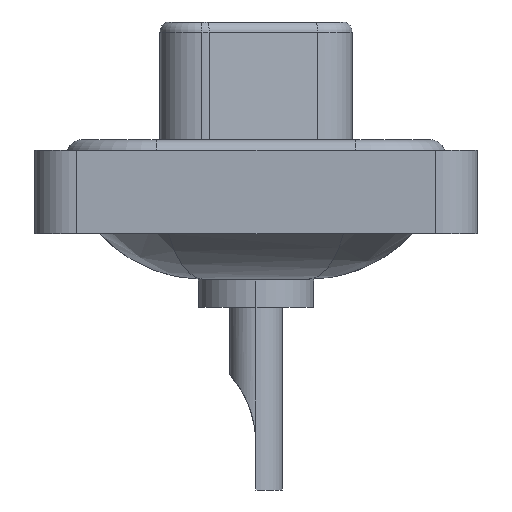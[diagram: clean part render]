
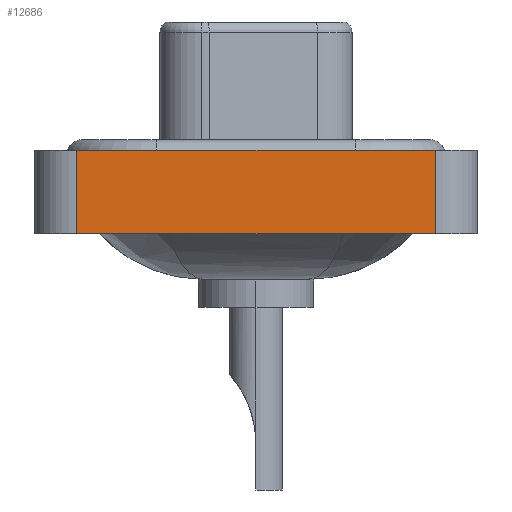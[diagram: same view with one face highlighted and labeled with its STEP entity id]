
A CAD part, left-side view. The second image highlights one B-rep face of the part: STEP entity #12686.
In plain terms, the highlighted planar face has unit normal (-1, 0, 0).
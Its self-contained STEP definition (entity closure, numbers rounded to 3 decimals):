
#684 = EDGE_CURVE ( 'NONE', #8553, #4325, #3760, .T. ) ;
#917 = EDGE_CURVE ( 'NONE', #8553, #6550, #10787, .T. ) ;
#930 = ORIENTED_EDGE ( 'NONE', *, *, #1071, .F. ) ;
#1071 = EDGE_CURVE ( 'NONE', #6550, #2067, #12765, .T. ) ;
#1132 = VECTOR ( 'NONE', #14625, 1000. ) ;
#2000 = CARTESIAN_POINT ( 'NONE',  ( -7.25, -8.55, 0.4 ) ) ;
#2067 = VERTEX_POINT ( 'NONE', #7733 ) ;
#2398 = AXIS2_PLACEMENT_3D ( 'NONE', #4824, #15515, #7355 ) ;
#2834 = LINE ( 'NONE', #7643, #1132 ) ;
#3626 = CARTESIAN_POINT ( 'NONE',  ( -7.25, 8.55, -3.6 ) ) ;
#3704 = DIRECTION ( 'NONE',  ( 0., 0., 1. ) ) ;
#3760 = LINE ( 'NONE', #14757, #11180 ) ;
#3839 = DIRECTION ( 'NONE',  ( 0., -1., 0. ) ) ;
#4325 = VERTEX_POINT ( 'NONE', #8404 ) ;
#4824 = CARTESIAN_POINT ( 'NONE',  ( -7.25, -8.55, -3.6 ) ) ;
#4906 = PLANE ( 'NONE',  #2398 ) ;
#6006 = FACE_OUTER_BOUND ( 'NONE', #14473, .T. ) ;
#6550 = VERTEX_POINT ( 'NONE', #6688 ) ;
#6558 = ORIENTED_EDGE ( 'NONE', *, *, #7739, .T. ) ;
#6688 = CARTESIAN_POINT ( 'NONE',  ( -7.25, 8.55, 0.4 ) ) ;
#6800 = DIRECTION ( 'NONE',  ( 0., -1., 0. ) ) ;
#6931 = ORIENTED_EDGE ( 'NONE', *, *, #917, .F. ) ;
#7131 = CARTESIAN_POINT ( 'NONE',  ( -7.25, 8.55, -3.6 ) ) ;
#7355 = DIRECTION ( 'NONE',  ( 0., 0., 1. ) ) ;
#7643 = CARTESIAN_POINT ( 'NONE',  ( -7.25, -8.55, -3.6 ) ) ;
#7733 = CARTESIAN_POINT ( 'NONE',  ( -7.25, -8.55, 0.4 ) ) ;
#7739 = EDGE_CURVE ( 'NONE', #4325, #2067, #2834, .T. ) ;
#8404 = CARTESIAN_POINT ( 'NONE',  ( -7.25, -8.55, -3.6 ) ) ;
#8553 = VERTEX_POINT ( 'NONE', #7131 ) ;
#10787 = LINE ( 'NONE', #3626, #14949 ) ;
#11180 = VECTOR ( 'NONE', #3839, 1000. ) ;
#12686 = ADVANCED_FACE ( 'NONE', ( #6006 ), #4906, .T. ) ;
#12765 = LINE ( 'NONE', #2000, #13443 ) ;
#12935 = ORIENTED_EDGE ( 'NONE', *, *, #684, .T. ) ;
#13443 = VECTOR ( 'NONE', #6800, 1000. ) ;
#14473 = EDGE_LOOP ( 'NONE', ( #6558, #930, #6931, #12935 ) ) ;
#14625 = DIRECTION ( 'NONE',  ( 0., 0., 1. ) ) ;
#14757 = CARTESIAN_POINT ( 'NONE',  ( -7.25, -8.55, -3.6 ) ) ;
#14949 = VECTOR ( 'NONE', #3704, 1000. ) ;
#15515 = DIRECTION ( 'NONE',  ( -1., 0., 0. ) ) ;
